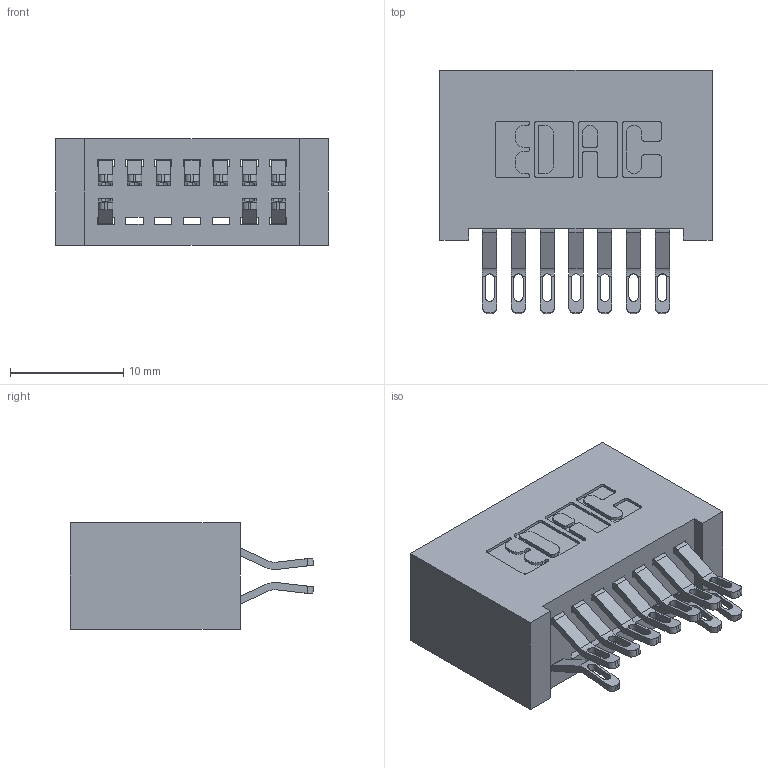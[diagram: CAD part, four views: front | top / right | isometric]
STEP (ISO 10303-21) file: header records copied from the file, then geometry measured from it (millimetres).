
FILE_DESCRIPTION (( 'STEP AP203' ), '1' );
FILE_NAME ('392-014-555-201.STEP', '2018-08-15T00:16:44', ( '' ), ( '' ), 'SwSTEP 2.0', 'SolidWorks 2016', '' );
FILE_SCHEMA (( 'CONFIG_CONTROL_DESIGN' ));
Length unit declared in the file: inch
Products named in the file (3): 342 Part_Lugless; 345-292-001_555 Tail; 392-014-555-201
Assembly tree (11 placements, depth 2):
  392-014-555-201
    342 Part_Lugless
    345-292-001_555 Tail  x10
Bounding box: 24.03 x 21.47 x 9.4 mm (x, y, z)
Volume: 2424.6 mm3; surface area: 3428.2 mm2
Topology: 11 solids, 11 shells, 706 faces, 2189 edges, 1458 vertices
Faces by surface type: plane 426, cylinder 280
Entity records: 8819 total; most frequent: CARTESIAN_POINT 1552, ORIENTED_EDGE 1462, DIRECTION 1347, EDGE_CURVE 731, LINE 591, VECTOR 591, VERTEX_POINT 486, AXIS2_PLACEMENT_3D 378
